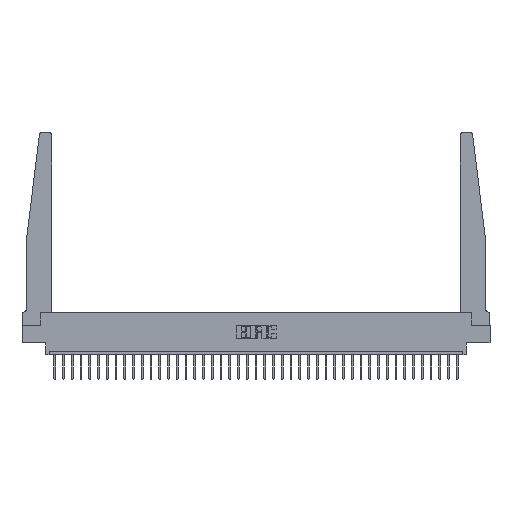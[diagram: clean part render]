
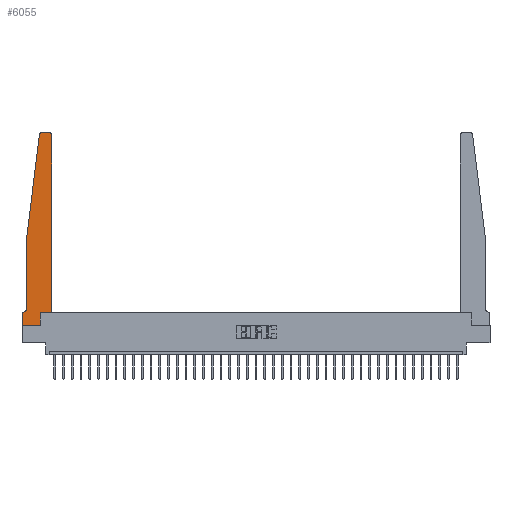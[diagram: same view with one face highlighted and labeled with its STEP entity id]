
A CAD part, top view. The second image highlights one B-rep face of the part: STEP entity #6055.
In plain terms, the highlighted planar face has unit normal (0, 0, 1).
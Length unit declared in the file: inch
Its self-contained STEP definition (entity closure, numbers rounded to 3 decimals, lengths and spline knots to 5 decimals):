
#310 = CARTESIAN_POINT ( 'NONE',  ( 0.065, 0.1875, 0.37 ) ) ;
#510 = CARTESIAN_POINT ( 'NONE',  ( 0.27653, 2.75, 0.37 ) ) ;
#640 = AXIS2_PLACEMENT_3D ( 'NONE', #23202, #11148, #23366 ) ;
#1502 = DIRECTION ( 'NONE',  ( 1., 0., 0. ) ) ;
#2027 = CARTESIAN_POINT ( 'NONE',  ( 0.395, 2.75, 0.37 ) ) ;
#2285 = CARTESIAN_POINT ( 'NONE',  ( 0.24675, 2.72367, 0.37 ) ) ;
#2344 = DIRECTION ( 'NONE',  ( 0., 0., 1. ) ) ;
#2869 = VERTEX_POINT ( 'NONE', #2285 ) ;
#2911 = CARTESIAN_POINT ( 'NONE',  ( 0.25, 2.75, 0.37 ) ) ;
#2978 = LINE ( 'NONE', #21655, #16624 ) ;
#3138 = EDGE_CURVE ( 'NONE', #9220, #13724, #12034, .T. ) ;
#3284 = VERTEX_POINT ( 'NONE', #22657 ) ;
#3805 = DIRECTION ( 'NONE',  ( 1., 0., 0. ) ) ;
#4432 = FACE_OUTER_BOUND ( 'NONE', #17547, .T. ) ;
#4486 = CIRCLE ( 'NONE', #640, 0.03 ) ;
#5288 = LINE ( 'NONE', #310, #26589 ) ;
#5788 = EDGE_CURVE ( 'NONE', #24680, #21467, #25708, .T. ) ;
#6055 = ADVANCED_FACE ( 'NONE', ( #4432 ), #25007, .T. ) ;
#6409 = ORIENTED_EDGE ( 'NONE', *, *, #17451, .T. ) ;
#7497 = VERTEX_POINT ( 'NONE', #23829 ) ;
#9179 = LINE ( 'NONE', #32964, #17311 ) ;
#9220 = VERTEX_POINT ( 'NONE', #20409 ) ;
#9406 = DIRECTION ( 'NONE',  ( -1., 0., 0. ) ) ;
#9532 = DIRECTION ( 'NONE',  ( 0., 1., 0. ) ) ;
#9858 = CARTESIAN_POINT ( 'NONE',  ( 0., 0., 0.37 ) ) ;
#9984 = CARTESIAN_POINT ( 'NONE',  ( 0.2605, 0., 0.37 ) ) ;
#10254 = VERTEX_POINT ( 'NONE', #29532 ) ;
#10594 = DIRECTION ( 'NONE',  ( 1., 0., 0. ) ) ;
#10781 = DIRECTION ( 'NONE',  ( -1., 0., 0. ) ) ;
#11015 = VECTOR ( 'NONE', #33572, 39.37008 ) ;
#11039 = ORIENTED_EDGE ( 'NONE', *, *, #5788, .T. ) ;
#11148 = DIRECTION ( 'NONE',  ( 0., 0., 1. ) ) ;
#11561 = VECTOR ( 'NONE', #3805, 39.37008 ) ;
#12034 = LINE ( 'NONE', #16824, #11561 ) ;
#12326 = CARTESIAN_POINT ( 'NONE',  ( 0., 0.1875, 0.37 ) ) ;
#13019 = VERTEX_POINT ( 'NONE', #23797 ) ;
#13055 = EDGE_CURVE ( 'NONE', #7497, #3284, #5288, .T. ) ;
#13724 = VERTEX_POINT ( 'NONE', #9984 ) ;
#14696 = DIRECTION ( 'NONE',  ( 1., 0., 0. ) ) ;
#14855 = EDGE_CURVE ( 'NONE', #23845, #27940, #21694, .T. ) ;
#15204 = LINE ( 'NONE', #17268, #21824 ) ;
#15695 = ORIENTED_EDGE ( 'NONE', *, *, #16962, .T. ) ;
#16538 = DIRECTION ( 'NONE',  ( 0., -1., 0. ) ) ;
#16624 = VECTOR ( 'NONE', #29511, 39.37008 ) ;
#16824 = CARTESIAN_POINT ( 'NONE',  ( 0., 0., 0.37 ) ) ;
#16921 = VECTOR ( 'NONE', #17563, 39.37008 ) ;
#16962 = EDGE_CURVE ( 'NONE', #27629, #13019, #15204, .T. ) ;
#17037 = EDGE_CURVE ( 'NONE', #27940, #7497, #24055, .T. ) ;
#17268 = CARTESIAN_POINT ( 'NONE',  ( 0.425, 0.18, 0.37 ) ) ;
#17311 = VECTOR ( 'NONE', #9532, 39.37008 ) ;
#17451 = EDGE_CURVE ( 'NONE', #3284, #9220, #20148, .T. ) ;
#17547 = EDGE_LOOP ( 'NONE', ( #11039, #23174, #20038, #30338, #26917, #28946, #6409, #28017, #26422, #15695, #23644, #24900 ) ) ;
#17563 = DIRECTION ( 'NONE',  ( 0., -1., 0. ) ) ;
#18602 = CARTESIAN_POINT ( 'NONE',  ( 0.065, 0.2375, 0.37 ) ) ;
#20038 = ORIENTED_EDGE ( 'NONE', *, *, #28464, .T. ) ;
#20131 = CARTESIAN_POINT ( 'NONE',  ( 0.065, 1.25, 0.37 ) ) ;
#20148 = LINE ( 'NONE', #9858, #16921 ) ;
#20409 = CARTESIAN_POINT ( 'NONE',  ( 0., 0., 0.37 ) ) ;
#20729 = CARTESIAN_POINT ( 'NONE',  ( 0.2605, 0.18, 0.37 ) ) ;
#20897 = AXIS2_PLACEMENT_3D ( 'NONE', #12326, #33193, #1502 ) ;
#21310 = CIRCLE ( 'NONE', #24043, 0.03 ) ;
#21467 = VERTEX_POINT ( 'NONE', #510 ) ;
#21469 = EDGE_CURVE ( 'NONE', #10254, #24680, #4486, .T. ) ;
#21655 = CARTESIAN_POINT ( 'NONE',  ( 0.425, 0.18, 0.37 ) ) ;
#21684 = VECTOR ( 'NONE', #29812, 39.37008 ) ;
#21694 = LINE ( 'NONE', #32120, #25837 ) ;
#21768 = LINE ( 'NONE', #29971, #21684 ) ;
#21824 = VECTOR ( 'NONE', #14696, 39.37008 ) ;
#22657 = CARTESIAN_POINT ( 'NONE',  ( 0., 0.1875, 0.37 ) ) ;
#22913 = CARTESIAN_POINT ( 'NONE',  ( 0.015, 0.2375, 0.37 ) ) ;
#23174 = ORIENTED_EDGE ( 'NONE', *, *, #29964, .T. ) ;
#23202 = CARTESIAN_POINT ( 'NONE',  ( 0.395, 2.72, 0.37 ) ) ;
#23270 = CARTESIAN_POINT ( 'NONE',  ( 0.27653, 2.72, 0.37 ) ) ;
#23366 = DIRECTION ( 'NONE',  ( 1., 0., 0. ) ) ;
#23644 = ORIENTED_EDGE ( 'NONE', *, *, #25648, .T. ) ;
#23797 = CARTESIAN_POINT ( 'NONE',  ( 0.425, 0.18, 0.37 ) ) ;
#23829 = CARTESIAN_POINT ( 'NONE',  ( 0.015, 0.1875, 0.37 ) ) ;
#23845 = VERTEX_POINT ( 'NONE', #20131 ) ;
#24043 = AXIS2_PLACEMENT_3D ( 'NONE', #23270, #2344, #10594 ) ;
#24055 = CIRCLE ( 'NONE', #26771, 0.05 ) ;
#24680 = VERTEX_POINT ( 'NONE', #2027 ) ;
#24900 = ORIENTED_EDGE ( 'NONE', *, *, #21469, .T. ) ;
#25007 = PLANE ( 'NONE',  #20897 ) ;
#25648 = EDGE_CURVE ( 'NONE', #13019, #10254, #2978, .T. ) ;
#25708 = LINE ( 'NONE', #2911, #11015 ) ;
#25837 = VECTOR ( 'NONE', #16538, 39.37008 ) ;
#26422 = ORIENTED_EDGE ( 'NONE', *, *, #29000, .T. ) ;
#26589 = VECTOR ( 'NONE', #10781, 39.37008 ) ;
#26771 = AXIS2_PLACEMENT_3D ( 'NONE', #22913, #30284, #9406 ) ;
#26917 = ORIENTED_EDGE ( 'NONE', *, *, #17037, .T. ) ;
#27629 = VERTEX_POINT ( 'NONE', #20729 ) ;
#27940 = VERTEX_POINT ( 'NONE', #18602 ) ;
#28017 = ORIENTED_EDGE ( 'NONE', *, *, #3138, .T. ) ;
#28464 = EDGE_CURVE ( 'NONE', #2869, #23845, #21768, .T. ) ;
#28946 = ORIENTED_EDGE ( 'NONE', *, *, #13055, .T. ) ;
#29000 = EDGE_CURVE ( 'NONE', #13724, #27629, #9179, .T. ) ;
#29511 = DIRECTION ( 'NONE',  ( 0., 1., 0. ) ) ;
#29532 = CARTESIAN_POINT ( 'NONE',  ( 0.425, 2.72, 0.37 ) ) ;
#29812 = DIRECTION ( 'NONE',  ( -0.122, -0.992, 0. ) ) ;
#29964 = EDGE_CURVE ( 'NONE', #21467, #2869, #21310, .T. ) ;
#29971 = CARTESIAN_POINT ( 'NONE',  ( 0.065, 1.25, 0.37 ) ) ;
#30284 = DIRECTION ( 'NONE',  ( 0., 0., -1. ) ) ;
#30338 = ORIENTED_EDGE ( 'NONE', *, *, #14855, .T. ) ;
#32120 = CARTESIAN_POINT ( 'NONE',  ( 0.065, 1.25, 0.37 ) ) ;
#32964 = CARTESIAN_POINT ( 'NONE',  ( 0.2605, 0.18, 0.37 ) ) ;
#33193 = DIRECTION ( 'NONE',  ( 0., 0., 1. ) ) ;
#33572 = DIRECTION ( 'NONE',  ( -1., 0., 0. ) ) ;
